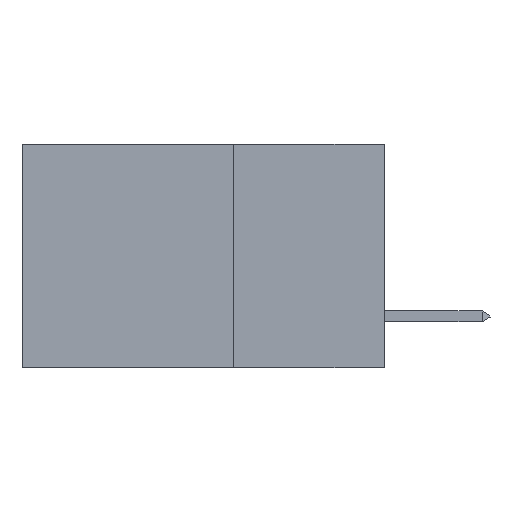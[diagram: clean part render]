
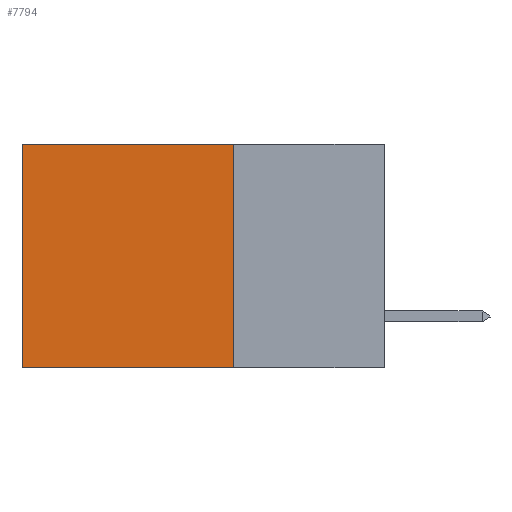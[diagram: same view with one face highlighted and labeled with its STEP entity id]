
A CAD part, left-side view. The second image highlights one B-rep face of the part: STEP entity #7794.
In plain terms, the highlighted planar face has unit normal (-1, 0, 0).
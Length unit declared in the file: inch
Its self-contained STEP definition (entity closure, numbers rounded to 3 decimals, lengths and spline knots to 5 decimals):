
#95 = EDGE_CURVE ( 'NONE', #4074, #6944, #5890, .T. ) ;
#484 = LINE ( 'NONE', #3809, #6854 ) ;
#622 = CARTESIAN_POINT ( 'NONE',  ( 0.2875, 0.6, -0.37 ) ) ;
#932 = CARTESIAN_POINT ( 'NONE',  ( 0.2875, 0.25, 0. ) ) ;
#1314 = DIRECTION ( 'NONE',  ( 0., 1., 0. ) ) ;
#1569 = CARTESIAN_POINT ( 'NONE',  ( 0.2875, 0.25, -0.37 ) ) ;
#1689 = VECTOR ( 'NONE', #3197, 39.37008 ) ;
#1872 = CARTESIAN_POINT ( 'NONE',  ( 0.2875, 0.25, 0. ) ) ;
#3035 = CARTESIAN_POINT ( 'NONE',  ( 0.2875, 0.6, 0. ) ) ;
#3197 = DIRECTION ( 'NONE',  ( 0., 1., 0. ) ) ;
#3809 = CARTESIAN_POINT ( 'NONE',  ( 0.2875, 0.25, 0. ) ) ;
#4074 = VERTEX_POINT ( 'NONE', #932 ) ;
#5571 = LINE ( 'NONE', #6721, #1689 ) ;
#5890 = LINE ( 'NONE', #7202, #10187 ) ;
#6311 = VECTOR ( 'NONE', #8037, 39.37008 ) ;
#6350 = CARTESIAN_POINT ( 'NONE',  ( 0.2875, 0.6, 0. ) ) ;
#6458 = EDGE_LOOP ( 'NONE', ( #10702, #10348, #10598, #9802 ) ) ;
#6721 = CARTESIAN_POINT ( 'NONE',  ( 0.2875, 0.25, -0.37 ) ) ;
#6854 = VECTOR ( 'NONE', #1314, 39.37008 ) ;
#6944 = VERTEX_POINT ( 'NONE', #1569 ) ;
#7202 = CARTESIAN_POINT ( 'NONE',  ( 0.2875, 0.25, 0. ) ) ;
#7794 = ADVANCED_FACE ( 'NONE', ( #10183 ), #8939, .F. ) ;
#8037 = DIRECTION ( 'NONE',  ( 0., 0., -1. ) ) ;
#8056 = EDGE_CURVE ( 'NONE', #4074, #8352, #484, .T. ) ;
#8249 = DIRECTION ( 'NONE',  ( 0., 0., -1. ) ) ;
#8352 = VERTEX_POINT ( 'NONE', #3035 ) ;
#8517 = LINE ( 'NONE', #6350, #6311 ) ;
#8939 = PLANE ( 'NONE',  #10330 ) ;
#8973 = DIRECTION ( 'NONE',  ( 0., 0., -1. ) ) ;
#9416 = EDGE_CURVE ( 'NONE', #8352, #10589, #8517, .T. ) ;
#9753 = DIRECTION ( 'NONE',  ( 1., 0., 0. ) ) ;
#9802 = ORIENTED_EDGE ( 'NONE', *, *, #8056, .T. ) ;
#10183 = FACE_OUTER_BOUND ( 'NONE', #6458, .T. ) ;
#10187 = VECTOR ( 'NONE', #8249, 39.37008 ) ;
#10330 = AXIS2_PLACEMENT_3D ( 'NONE', #1872, #9753, #8973 ) ;
#10348 = ORIENTED_EDGE ( 'NONE', *, *, #10563, .F. ) ;
#10563 = EDGE_CURVE ( 'NONE', #6944, #10589, #5571, .T. ) ;
#10589 = VERTEX_POINT ( 'NONE', #622 ) ;
#10598 = ORIENTED_EDGE ( 'NONE', *, *, #95, .F. ) ;
#10702 = ORIENTED_EDGE ( 'NONE', *, *, #9416, .T. ) ;
